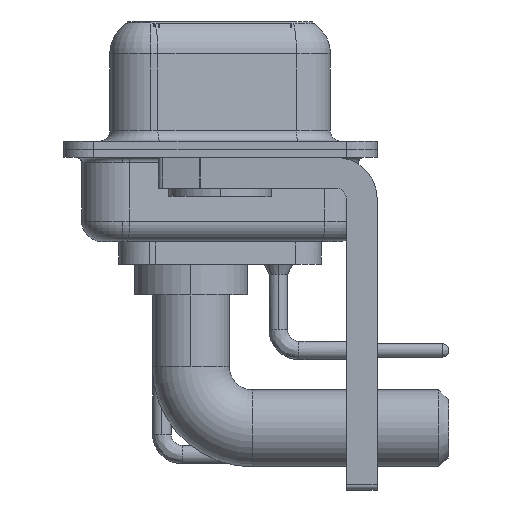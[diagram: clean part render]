
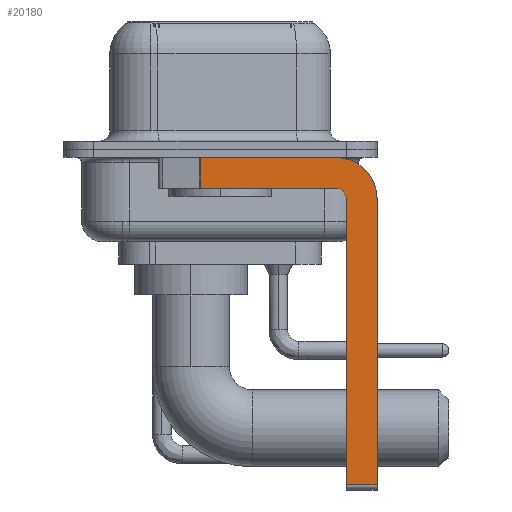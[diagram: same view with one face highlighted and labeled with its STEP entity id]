
A CAD part, left-side view. The second image highlights one B-rep face of the part: STEP entity #20180.
In plain terms, the highlighted planar face has unit normal (-1, 0, 0).
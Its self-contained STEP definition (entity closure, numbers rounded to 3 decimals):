
#37 = CARTESIAN_POINT ( 'NONE',  ( -2.9, -7.65, -2.4 ) ) ;
#486 = DIRECTION ( 'NONE',  ( 0., 1., 0. ) ) ;
#761 = VECTOR ( 'NONE', #22633, 1000. ) ;
#1146 = CARTESIAN_POINT ( 'NONE',  ( -2.9, 0.978, -1.9 ) ) ;
#2324 = DIRECTION ( 'NONE',  ( 1., 0., 0. ) ) ;
#2454 = LINE ( 'NONE', #7021, #5428 ) ;
#2520 = VECTOR ( 'NONE', #8906, 1000. ) ;
#2827 = DIRECTION ( 'NONE',  ( 0., 0., -1. ) ) ;
#2990 = ORIENTED_EDGE ( 'NONE', *, *, #4965, .F. ) ;
#3164 = DIRECTION ( 'NONE',  ( 0., 0., -1. ) ) ;
#4015 = LINE ( 'NONE', #24855, #9586 ) ;
#4965 = EDGE_CURVE ( 'NONE', #24070, #29073, #4015, .T. ) ;
#5428 = VECTOR ( 'NONE', #486, 1000. ) ;
#5559 = AXIS2_PLACEMENT_3D ( 'NONE', #25451, #2324, #6434 ) ;
#5882 = ORIENTED_EDGE ( 'NONE', *, *, #28699, .F. ) ;
#6270 = VERTEX_POINT ( 'NONE', #20006 ) ;
#6434 = DIRECTION ( 'NONE',  ( 0., 0., -1. ) ) ;
#7021 = CARTESIAN_POINT ( 'NONE',  ( -2.9, -5.65, -1.9 ) ) ;
#7186 = CARTESIAN_POINT ( 'NONE',  ( -2.9, -7.65, -16.35 ) ) ;
#7508 = ORIENTED_EDGE ( 'NONE', *, *, #24112, .F. ) ;
#7729 = EDGE_LOOP ( 'NONE', ( #8534, #20769, #7508, #26422, #5882, #19610, #2990, #24330 ) ) ;
#8534 = ORIENTED_EDGE ( 'NONE', *, *, #18030, .F. ) ;
#8906 = DIRECTION ( 'NONE',  ( 0., -1., 0. ) ) ;
#9586 = VECTOR ( 'NONE', #29752, 1000. ) ;
#10742 = CARTESIAN_POINT ( 'NONE',  ( -2.9, -5.65, -16.35 ) ) ;
#10767 = CIRCLE ( 'NONE', #22908, 2. ) ;
#12138 = EDGE_CURVE ( 'NONE', #13671, #18636, #16231, .T. ) ;
#12526 = AXIS2_PLACEMENT_3D ( 'NONE', #23625, #23922, #21343 ) ;
#12562 = CARTESIAN_POINT ( 'NONE',  ( -2.9, 0.978, -0.4 ) ) ;
#12783 = EDGE_CURVE ( 'NONE', #6270, #27227, #14959, .T. ) ;
#13671 = VERTEX_POINT ( 'NONE', #12562 ) ;
#13882 = PLANE ( 'NONE',  #5559 ) ;
#14850 = DIRECTION ( 'NONE',  ( 0., -1., 0. ) ) ;
#14959 = CIRCLE ( 'NONE', #12526, 0.5 ) ;
#16231 = LINE ( 'NONE', #25807, #27067 ) ;
#16434 = EDGE_CURVE ( 'NONE', #24670, #29073, #29168, .T. ) ;
#17334 = CARTESIAN_POINT ( 'NONE',  ( -2.9, -5.65, -2.4 ) ) ;
#17447 = VERTEX_POINT ( 'NONE', #28910 ) ;
#18030 = EDGE_CURVE ( 'NONE', #13671, #17447, #20468, .T. ) ;
#18379 = CARTESIAN_POINT ( 'NONE',  ( -2.9, -6.15, -16.6 ) ) ;
#18636 = VERTEX_POINT ( 'NONE', #1146 ) ;
#19610 = ORIENTED_EDGE ( 'NONE', *, *, #16434, .T. ) ;
#20006 = CARTESIAN_POINT ( 'NONE',  ( -2.9, -6.15, -2.4 ) ) ;
#20180 = ADVANCED_FACE ( 'NONE', ( #20435 ), #13882, .F. ) ;
#20435 = FACE_OUTER_BOUND ( 'NONE', #7729, .T. ) ;
#20468 = LINE ( 'NONE', #29781, #2520 ) ;
#20650 = LINE ( 'NONE', #18379, #761 ) ;
#20769 = ORIENTED_EDGE ( 'NONE', *, *, #12138, .T. ) ;
#21343 = DIRECTION ( 'NONE',  ( 0., 0., 1. ) ) ;
#22633 = DIRECTION ( 'NONE',  ( 0., 0., 1. ) ) ;
#22908 = AXIS2_PLACEMENT_3D ( 'NONE', #17334, #24008, #3164 ) ;
#23462 = EDGE_CURVE ( 'NONE', #17447, #24070, #10767, .T. ) ;
#23625 = CARTESIAN_POINT ( 'NONE',  ( -2.9, -5.65, -2.4 ) ) ;
#23922 = DIRECTION ( 'NONE',  ( -1., 0., 0. ) ) ;
#24008 = DIRECTION ( 'NONE',  ( 1., 0., 0. ) ) ;
#24070 = VERTEX_POINT ( 'NONE', #37 ) ;
#24112 = EDGE_CURVE ( 'NONE', #27227, #18636, #2454, .T. ) ;
#24330 = ORIENTED_EDGE ( 'NONE', *, *, #23462, .F. ) ;
#24670 = VERTEX_POINT ( 'NONE', #28140 ) ;
#24855 = CARTESIAN_POINT ( 'NONE',  ( -2.9, -7.65, -2.4 ) ) ;
#25451 = CARTESIAN_POINT ( 'NONE',  ( -2.9, -5.65, -2.4 ) ) ;
#25637 = CARTESIAN_POINT ( 'NONE',  ( -2.9, -5.65, -1.9 ) ) ;
#25807 = CARTESIAN_POINT ( 'NONE',  ( -2.9, 0.978, -1.9 ) ) ;
#26422 = ORIENTED_EDGE ( 'NONE', *, *, #12783, .F. ) ;
#27067 = VECTOR ( 'NONE', #2827, 1000. ) ;
#27227 = VERTEX_POINT ( 'NONE', #25637 ) ;
#28140 = CARTESIAN_POINT ( 'NONE',  ( -2.9, -6.15, -16.35 ) ) ;
#28699 = EDGE_CURVE ( 'NONE', #24670, #6270, #20650, .T. ) ;
#28910 = CARTESIAN_POINT ( 'NONE',  ( -2.9, -5.65, -0.4 ) ) ;
#29073 = VERTEX_POINT ( 'NONE', #7186 ) ;
#29168 = LINE ( 'NONE', #10742, #29759 ) ;
#29752 = DIRECTION ( 'NONE',  ( 0., 0., -1. ) ) ;
#29759 = VECTOR ( 'NONE', #14850, 1000. ) ;
#29781 = CARTESIAN_POINT ( 'NONE',  ( -2.9, 3., -0.4 ) ) ;
